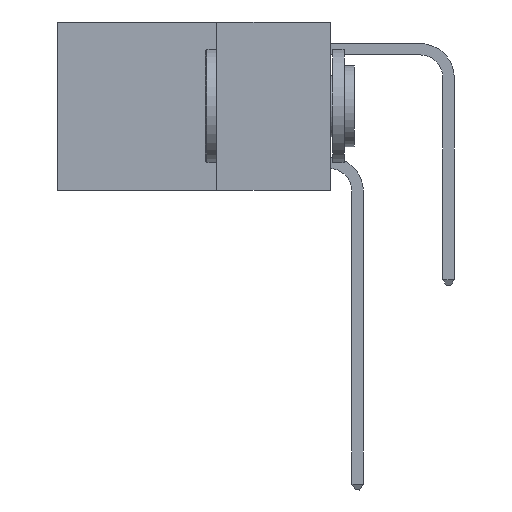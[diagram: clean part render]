
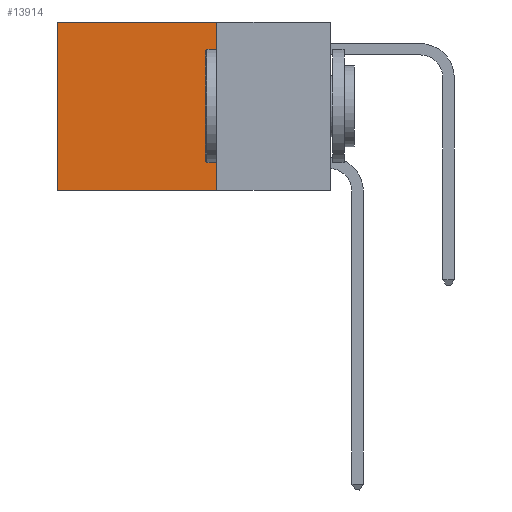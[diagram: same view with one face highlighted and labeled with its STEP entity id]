
A CAD part, left-side view. The second image highlights one B-rep face of the part: STEP entity #13914.
In plain terms, the highlighted planar face has unit normal (-1, 0, 0).
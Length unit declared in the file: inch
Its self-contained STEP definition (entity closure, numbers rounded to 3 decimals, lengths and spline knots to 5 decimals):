
#99 = VERTEX_POINT ( 'NONE', #14251 ) ;
#662 = DIRECTION ( 'NONE',  ( 0., 0., -1. ) ) ;
#1157 = VECTOR ( 'NONE', #8622, 39.37008 ) ;
#1552 = LINE ( 'NONE', #7371, #1157 ) ;
#1819 = CARTESIAN_POINT ( 'NONE',  ( 0.2625, 0.25, -0.37 ) ) ;
#2850 = VERTEX_POINT ( 'NONE', #1819 ) ;
#4653 = LINE ( 'NONE', #14206, #5043 ) ;
#4812 = EDGE_CURVE ( 'NONE', #2850, #5084, #8143, .T. ) ;
#5043 = VECTOR ( 'NONE', #11827, 39.37008 ) ;
#5084 = VERTEX_POINT ( 'NONE', #15144 ) ;
#5179 = ORIENTED_EDGE ( 'NONE', *, *, #7346, .T. ) ;
#5271 = ORIENTED_EDGE ( 'NONE', *, *, #4812, .F. ) ;
#5474 = ORIENTED_EDGE ( 'NONE', *, *, #13390, .F. ) ;
#5491 = EDGE_LOOP ( 'NONE', ( #5179, #5271, #5474, #5509 ) ) ;
#5509 = ORIENTED_EDGE ( 'NONE', *, *, #7327, .T. ) ;
#6144 = CARTESIAN_POINT ( 'NONE',  ( 0.2625, 0.6, 0. ) ) ;
#6803 = FACE_OUTER_BOUND ( 'NONE', #5491, .T. ) ;
#6984 = CARTESIAN_POINT ( 'NONE',  ( 0.2625, 0.25, 0. ) ) ;
#7327 = EDGE_CURVE ( 'NONE', #99, #14382, #1552, .T. ) ;
#7346 = EDGE_CURVE ( 'NONE', #14382, #5084, #10734, .T. ) ;
#7371 = CARTESIAN_POINT ( 'NONE',  ( 0.2625, 0.25, 0. ) ) ;
#7480 = VECTOR ( 'NONE', #11067, 39.37008 ) ;
#8143 = LINE ( 'NONE', #11129, #14194 ) ;
#8224 = DIRECTION ( 'NONE',  ( 1., 0., 0. ) ) ;
#8622 = DIRECTION ( 'NONE',  ( 0., 1., 0. ) ) ;
#8746 = DIRECTION ( 'NONE',  ( 0., 1., 0. ) ) ;
#10734 = LINE ( 'NONE', #6144, #7480 ) ;
#11067 = DIRECTION ( 'NONE',  ( 0., 0., -1. ) ) ;
#11129 = CARTESIAN_POINT ( 'NONE',  ( 0.2625, 0.25, -0.37 ) ) ;
#11827 = DIRECTION ( 'NONE',  ( 0., 0., -1. ) ) ;
#12692 = CARTESIAN_POINT ( 'NONE',  ( 0.2625, 0.6, 0. ) ) ;
#13390 = EDGE_CURVE ( 'NONE', #99, #2850, #4653, .T. ) ;
#13914 = ADVANCED_FACE ( 'NONE', ( #6803 ), #15362, .F. ) ;
#14194 = VECTOR ( 'NONE', #8746, 39.37008 ) ;
#14206 = CARTESIAN_POINT ( 'NONE',  ( 0.2625, 0.25, 0. ) ) ;
#14251 = CARTESIAN_POINT ( 'NONE',  ( 0.2625, 0.25, 0. ) ) ;
#14382 = VERTEX_POINT ( 'NONE', #12692 ) ;
#14487 = AXIS2_PLACEMENT_3D ( 'NONE', #6984, #8224, #662 ) ;
#15144 = CARTESIAN_POINT ( 'NONE',  ( 0.2625, 0.6, -0.37 ) ) ;
#15362 = PLANE ( 'NONE',  #14487 ) ;
